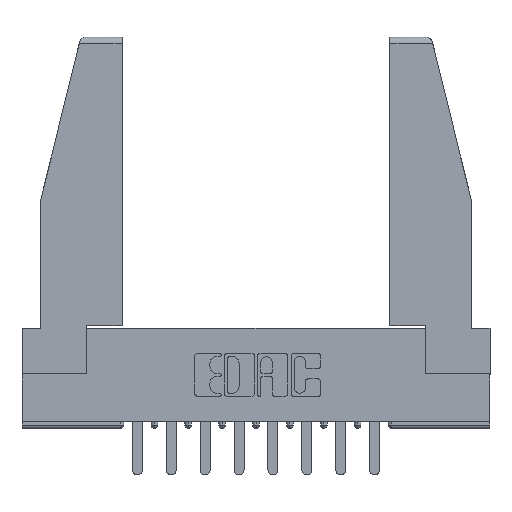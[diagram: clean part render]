
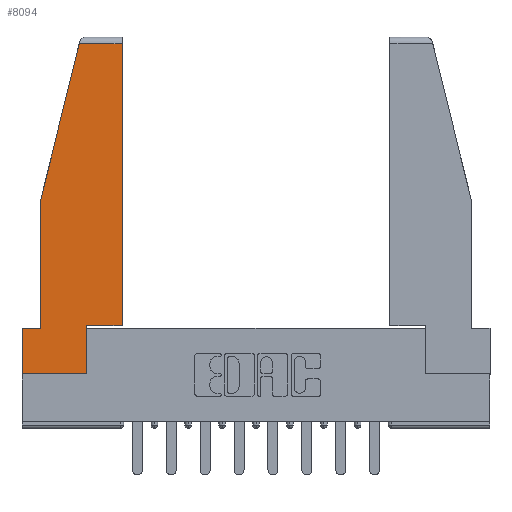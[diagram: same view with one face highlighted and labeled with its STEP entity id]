
A CAD part, top view. The second image highlights one B-rep face of the part: STEP entity #8094.
In plain terms, the highlighted planar face has unit normal (0, 0, 1).
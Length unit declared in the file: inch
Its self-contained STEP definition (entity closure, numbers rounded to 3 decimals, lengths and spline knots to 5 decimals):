
#68 = ORIENTED_EDGE ( 'NONE', *, *, #12018, .T. ) ;
#107 = VECTOR ( 'NONE', #14014, 39.37008 ) ;
#241 = VERTEX_POINT ( 'NONE', #12211 ) ;
#407 = LINE ( 'NONE', #4797, #12470 ) ;
#543 = ORIENTED_EDGE ( 'NONE', *, *, #12228, .T. ) ;
#842 = ORIENTED_EDGE ( 'NONE', *, *, #10260, .T. ) ;
#1127 = LINE ( 'NONE', #3433, #8613 ) ;
#1395 = PLANE ( 'NONE',  #4624 ) ;
#2238 = ORIENTED_EDGE ( 'NONE', *, *, #9749, .T. ) ;
#2423 = CARTESIAN_POINT ( 'NONE',  ( 0., 0., 0. ) ) ;
#2825 = VECTOR ( 'NONE', #7594, 39.37008 ) ;
#2896 = CARTESIAN_POINT ( 'NONE',  ( 0.086, 0.8, 0. ) ) ;
#2920 = CARTESIAN_POINT ( 'NONE',  ( 0., 0., 0. ) ) ;
#2933 = LINE ( 'NONE', #12900, #11431 ) ;
#2940 = VERTEX_POINT ( 'NONE', #9233 ) ;
#3433 = CARTESIAN_POINT ( 'NONE',  ( 0.297, 0.223, 0. ) ) ;
#3443 = ORIENTED_EDGE ( 'NONE', *, *, #4264, .T. ) ;
#3817 = LINE ( 'NONE', #7149, #107 ) ;
#3866 = DIRECTION ( 'NONE',  ( 0., -1., 0. ) ) ;
#4072 = DIRECTION ( 'NONE',  ( -0.239, -0.971, 0. ) ) ;
#4264 = EDGE_CURVE ( 'NONE', #9667, #11057, #407, .T. ) ;
#4432 = DIRECTION ( 'NONE',  ( 1., 0., 0. ) ) ;
#4486 = ORIENTED_EDGE ( 'NONE', *, *, #13935, .T. ) ;
#4562 = DIRECTION ( 'NONE',  ( 1., 0., 0. ) ) ;
#4624 = AXIS2_PLACEMENT_3D ( 'NONE', #8071, #6756, #5792 ) ;
#4664 = VECTOR ( 'NONE', #13148, 39.37008 ) ;
#4715 = FACE_OUTER_BOUND ( 'NONE', #12465, .T. ) ;
#4797 = CARTESIAN_POINT ( 'NONE',  ( 0., 0.21, 0. ) ) ;
#4944 = EDGE_CURVE ( 'NONE', #6917, #9667, #2933, .T. ) ;
#5229 = CARTESIAN_POINT ( 'NONE',  ( 0.271, 1.55, 0. ) ) ;
#5360 = LINE ( 'NONE', #13106, #6564 ) ;
#5792 = DIRECTION ( 'NONE',  ( 1., 0., 0. ) ) ;
#6244 = CARTESIAN_POINT ( 'NONE',  ( 0.461, 0.223, 0. ) ) ;
#6344 = ORIENTED_EDGE ( 'NONE', *, *, #9058, .T. ) ;
#6462 = DIRECTION ( 'NONE',  ( -1., 0., 0. ) ) ;
#6506 = CARTESIAN_POINT ( 'NONE',  ( 0.297, 0., 0. ) ) ;
#6564 = VECTOR ( 'NONE', #9795, 39.37008 ) ;
#6644 = VERTEX_POINT ( 'NONE', #8836 ) ;
#6756 = DIRECTION ( 'NONE',  ( 0., 0., 1. ) ) ;
#6917 = VERTEX_POINT ( 'NONE', #7329 ) ;
#6963 = LINE ( 'NONE', #2423, #14160 ) ;
#7149 = CARTESIAN_POINT ( 'NONE',  ( 0., 1.52, 0. ) ) ;
#7329 = CARTESIAN_POINT ( 'NONE',  ( 0.086, 0.21, 0. ) ) ;
#7383 = VERTEX_POINT ( 'NONE', #2896 ) ;
#7429 = LINE ( 'NONE', #5229, #8830 ) ;
#7594 = DIRECTION ( 'NONE',  ( 0., -1., 0. ) ) ;
#8071 = CARTESIAN_POINT ( 'NONE',  ( 0., 0., 0. ) ) ;
#8094 = ADVANCED_FACE ( 'NONE', ( #4715 ), #1395, .T. ) ;
#8613 = VECTOR ( 'NONE', #4432, 39.37008 ) ;
#8830 = VECTOR ( 'NONE', #4072, 39.37008 ) ;
#8836 = CARTESIAN_POINT ( 'NONE',  ( 0.461, 1.52, 0. ) ) ;
#9058 = EDGE_CURVE ( 'NONE', #2940, #13056, #1127, .T. ) ;
#9233 = CARTESIAN_POINT ( 'NONE',  ( 0.297, 0.223, 0. ) ) ;
#9482 = VERTEX_POINT ( 'NONE', #12590 ) ;
#9667 = VERTEX_POINT ( 'NONE', #9696 ) ;
#9696 = CARTESIAN_POINT ( 'NONE',  ( 0., 0.21, 0. ) ) ;
#9749 = EDGE_CURVE ( 'NONE', #241, #2940, #13016, .T. ) ;
#9795 = DIRECTION ( 'NONE',  ( 0., 1., 0. ) ) ;
#10238 = ORIENTED_EDGE ( 'NONE', *, *, #4944, .T. ) ;
#10260 = EDGE_CURVE ( 'NONE', #7383, #6917, #14282, .T. ) ;
#10371 = ORIENTED_EDGE ( 'NONE', *, *, #10621, .T. ) ;
#10621 = EDGE_CURVE ( 'NONE', #9482, #7383, #7429, .T. ) ;
#11057 = VERTEX_POINT ( 'NONE', #2920 ) ;
#11431 = VECTOR ( 'NONE', #6462, 39.37008 ) ;
#12018 = EDGE_CURVE ( 'NONE', #11057, #241, #6963, .T. ) ;
#12211 = CARTESIAN_POINT ( 'NONE',  ( 0.297, 0., 0. ) ) ;
#12228 = EDGE_CURVE ( 'NONE', #13056, #6644, #5360, .T. ) ;
#12465 = EDGE_LOOP ( 'NONE', ( #543, #4486, #10371, #842, #10238, #3443, #68, #2238, #6344 ) ) ;
#12470 = VECTOR ( 'NONE', #3866, 39.37008 ) ;
#12590 = CARTESIAN_POINT ( 'NONE',  ( 0.2636, 1.52, 0. ) ) ;
#12900 = CARTESIAN_POINT ( 'NONE',  ( 0., 0.21, 0. ) ) ;
#13016 = LINE ( 'NONE', #6506, #4664 ) ;
#13056 = VERTEX_POINT ( 'NONE', #6244 ) ;
#13070 = CARTESIAN_POINT ( 'NONE',  ( 0.086, 0.8, 0. ) ) ;
#13106 = CARTESIAN_POINT ( 'NONE',  ( 0.461, 0.223, 0. ) ) ;
#13148 = DIRECTION ( 'NONE',  ( 0., 1., 0. ) ) ;
#13935 = EDGE_CURVE ( 'NONE', #6644, #9482, #3817, .T. ) ;
#14014 = DIRECTION ( 'NONE',  ( -1., 0., 0. ) ) ;
#14160 = VECTOR ( 'NONE', #4562, 39.37008 ) ;
#14282 = LINE ( 'NONE', #13070, #2825 ) ;
